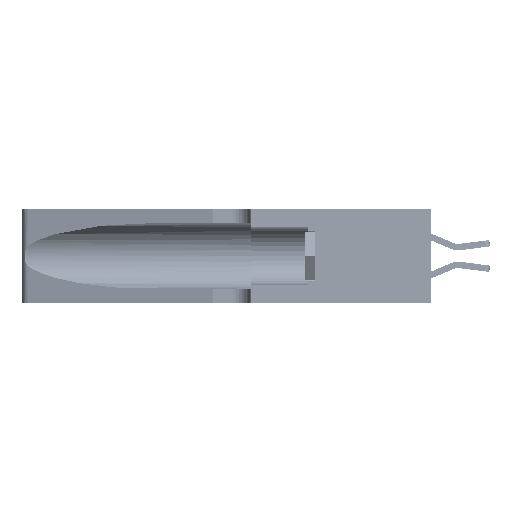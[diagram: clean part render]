
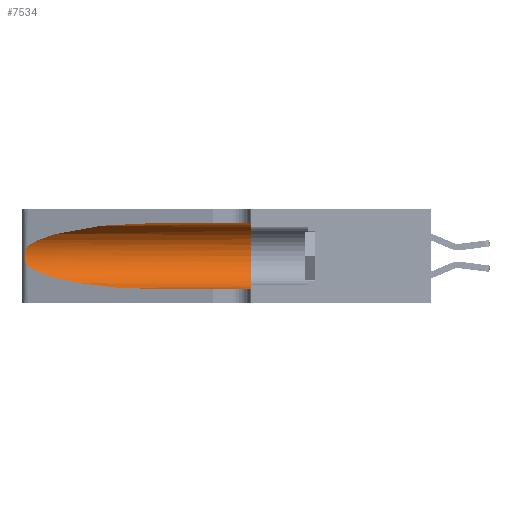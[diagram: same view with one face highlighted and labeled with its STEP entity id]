
A CAD part, left-side view. The second image highlights one B-rep face of the part: STEP entity #7534.
In plain terms, the highlighted cylindrical face has radius 3.308 mm (diameter 6.617 mm), a partial arc.
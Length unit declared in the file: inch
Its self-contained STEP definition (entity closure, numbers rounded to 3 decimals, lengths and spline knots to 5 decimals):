
#22 = EDGE_LOOP ( 'NONE', ( #4099, #16569, #32143, #16277, #2934, #26315 ) ) ;
#530 = CARTESIAN_POINT ( 'NONE',  ( 0.25487, 1.22718, 0.22369 ) ) ;
#740 = CARTESIAN_POINT ( 'NONE',  ( 0.18966, 0.96281, 0.31525 ) ) ;
#1247 = CARTESIAN_POINT ( 'NONE',  ( 0.25487, 1.22718, 0.14631 ) ) ;
#2065 = VERTEX_POINT ( 'NONE', #17837 ) ;
#2285 = B_SPLINE_CURVE_WITH_KNOTS ( 'NONE', 3,
 ( #17536, #35168, #6294, #12096, #32361, #14986, #35302, #17913, #7167, #18283, #29850, #21093, #12471, #1247 ),
 .UNSPECIFIED., .F., .F.,
 ( 4, 2, 2, 2, 2, 2, 4 ),
 ( 0., 0.00027, 0.00053, 0.00107, 0.0016, 0.00187, 0.00214 ),
 .UNSPECIFIED. ) ;
#2934 = ORIENTED_EDGE ( 'NONE', *, *, #25403, .F. ) ;
#4099 = ORIENTED_EDGE ( 'NONE', *, *, #23079, .T. ) ;
#4515 = CARTESIAN_POINT ( 'NONE',  ( 0.1305, 0.72297, 0.31525 ) ) ;
#4922 = VERTEX_POINT ( 'NONE', #14942 ) ;
#5073 = CARTESIAN_POINT ( 'NONE',  ( 0.18966, 0.96281, 0.05475 ) ) ;
#5209 = VECTOR ( 'NONE', #25267, 39.37008 ) ;
#6294 = CARTESIAN_POINT ( 'NONE',  ( 0.25639, 1.23184, 0.21858 ) ) ;
#6419 = CARTESIAN_POINT ( 'NONE',  ( 0.1305, 0.72297, 0.31525 ) ) ;
#7167 = CARTESIAN_POINT ( 'NONE',  ( 0.26017, 1.23833, 0.17102 ) ) ;
#7534 = ADVANCED_FACE ( 'NONE', ( #18487 ), #13539, .F. ) ;
#9606 = CARTESIAN_POINT ( 'NONE',  ( 0.2373, 1.15595, 0.28018 ) ) ;
#9680 = EDGE_CURVE ( 'NONE', #2065, #4922, #17294, .T. ) ;
#10621 = VERTEX_POINT ( 'NONE', #17409 ) ;
#12096 = CARTESIAN_POINT ( 'NONE',  ( 0.25787, 1.23484, 0.2124 ) ) ;
#12471 = CARTESIAN_POINT ( 'NONE',  ( 0.25555, 1.22993, 0.14849 ) ) ;
#13098 = CARTESIAN_POINT ( 'NONE',  ( 0.1305, 1.61858, 0.31525 ) ) ;
#13400 = CARTESIAN_POINT ( 'NONE',  ( 0.1305, 1.61858, 0.05475 ) ) ;
#13539 = CYLINDRICAL_SURFACE ( 'NONE', #31879, 0.13025 ) ;
#14942 = CARTESIAN_POINT ( 'NONE',  ( 0.1305, 0.72297, 0.05475 ) ) ;
#14986 = CARTESIAN_POINT ( 'NONE',  ( 0.26018, 1.23835, 0.19895 ) ) ;
#15150 = CARTESIAN_POINT ( 'NONE',  ( 0.1305, 0.35, 0.185 ) ) ;
#15264 = CARTESIAN_POINT ( 'NONE',  ( 0.25487, 1.22718, 0.22369 ) ) ;
#16277 = ORIENTED_EDGE ( 'NONE', *, *, #33490, .T. ) ;
#16569 = ORIENTED_EDGE ( 'NONE', *, *, #29735, .T. ) ;
#17294 =( BOUNDED_CURVE ( )  B_SPLINE_CURVE ( 3, ( #21756, #33416, #5073, #35165 ),
 .UNSPECIFIED., .F., .F. ) 
 B_SPLINE_CURVE_WITH_KNOTS ( ( 4, 4 ),
 ( 3.44316, 4.71239 ),
 .UNSPECIFIED. ) 
 CURVE ( )  GEOMETRIC_REPRESENTATION_ITEM ( )  RATIONAL_B_SPLINE_CURVE ( ( 1., 0.87, 0.87, 1. ) ) 
 REPRESENTATION_ITEM ( '' )  );
#17409 = CARTESIAN_POINT ( 'NONE',  ( 0.1305, 0.35, 0.31525 ) ) ;
#17536 = CARTESIAN_POINT ( 'NONE',  ( 0.25487, 1.22718, 0.22369 ) ) ;
#17837 = CARTESIAN_POINT ( 'NONE',  ( 0.25487, 1.22718, 0.14631 ) ) ;
#17913 = CARTESIAN_POINT ( 'NONE',  ( 0.26075, 1.23896, 0.178 ) ) ;
#18175 = CARTESIAN_POINT ( 'NONE',  ( 0.1305, 0.35, 0.05475 ) ) ;
#18280 = LINE ( 'NONE', #13098, #5209 ) ;
#18283 = CARTESIAN_POINT ( 'NONE',  ( 0.25856, 1.23593, 0.16098 ) ) ;
#18487 = FACE_OUTER_BOUND ( 'NONE', #22, .T. ) ;
#20048 = LINE ( 'NONE', #13400, #34570 ) ;
#20100 =( BOUNDED_CURVE ( )  B_SPLINE_CURVE ( 3, ( #6419, #740, #9606, #15264 ),
 .UNSPECIFIED., .F., .T. ) 
 B_SPLINE_CURVE_WITH_KNOTS ( ( 4, 4 ),
 ( 1.5708, 2.84003 ),
 .UNSPECIFIED. ) 
 CURVE ( )  GEOMETRIC_REPRESENTATION_ITEM ( )  RATIONAL_B_SPLINE_CURVE ( ( 1., 0.87, 0.87, 1. ) ) 
 REPRESENTATION_ITEM ( '' )  );
#20379 = CARTESIAN_POINT ( 'NONE',  ( 0.1305, 1.61858, 0.185 ) ) ;
#20996 = DIRECTION ( 'NONE',  ( 0., 1., 0. ) ) ;
#21093 = CARTESIAN_POINT ( 'NONE',  ( 0.25639, 1.23186, 0.15144 ) ) ;
#21756 = CARTESIAN_POINT ( 'NONE',  ( 0.25487, 1.22718, 0.14631 ) ) ;
#23033 = DIRECTION ( 'NONE',  ( 0., 0., -1. ) ) ;
#23079 = EDGE_CURVE ( 'NONE', #31838, #29095, #20100, .T. ) ;
#25267 = DIRECTION ( 'NONE',  ( 0., -1., 0. ) ) ;
#25403 = EDGE_CURVE ( 'NONE', #10621, #28002, #28160, .T. ) ;
#26212 = DIRECTION ( 'NONE',  ( 0., -1., 0. ) ) ;
#26315 = ORIENTED_EDGE ( 'NONE', *, *, #32322, .F. ) ;
#28002 = VERTEX_POINT ( 'NONE', #18175 ) ;
#28126 = DIRECTION ( 'NONE',  ( 0., -1., 0. ) ) ;
#28160 = CIRCLE ( 'NONE', #32767, 0.13025 ) ;
#29095 = VERTEX_POINT ( 'NONE', #530 ) ;
#29735 = EDGE_CURVE ( 'NONE', #29095, #2065, #2285, .T. ) ;
#29850 = CARTESIAN_POINT ( 'NONE',  ( 0.25789, 1.23486, 0.15765 ) ) ;
#31838 = VERTEX_POINT ( 'NONE', #4515 ) ;
#31879 = AXIS2_PLACEMENT_3D ( 'NONE', #20379, #26212, #23033 ) ;
#32143 = ORIENTED_EDGE ( 'NONE', *, *, #9680, .T. ) ;
#32322 = EDGE_CURVE ( 'NONE', #31838, #10621, #18280, .T. ) ;
#32361 = CARTESIAN_POINT ( 'NONE',  ( 0.25854, 1.2359, 0.20912 ) ) ;
#32767 = AXIS2_PLACEMENT_3D ( 'NONE', #15150, #20996, #32775 ) ;
#32775 = DIRECTION ( 'NONE',  ( 0., 0., 1. ) ) ;
#33416 = CARTESIAN_POINT ( 'NONE',  ( 0.2373, 1.15595, 0.08982 ) ) ;
#33490 = EDGE_CURVE ( 'NONE', #4922, #28002, #20048, .T. ) ;
#34570 = VECTOR ( 'NONE', #28126, 39.37008 ) ;
#35165 = CARTESIAN_POINT ( 'NONE',  ( 0.1305, 0.72297, 0.05475 ) ) ;
#35168 = CARTESIAN_POINT ( 'NONE',  ( 0.25555, 1.22994, 0.2215 ) ) ;
#35302 = CARTESIAN_POINT ( 'NONE',  ( 0.26075, 1.23896, 0.19203 ) ) ;
